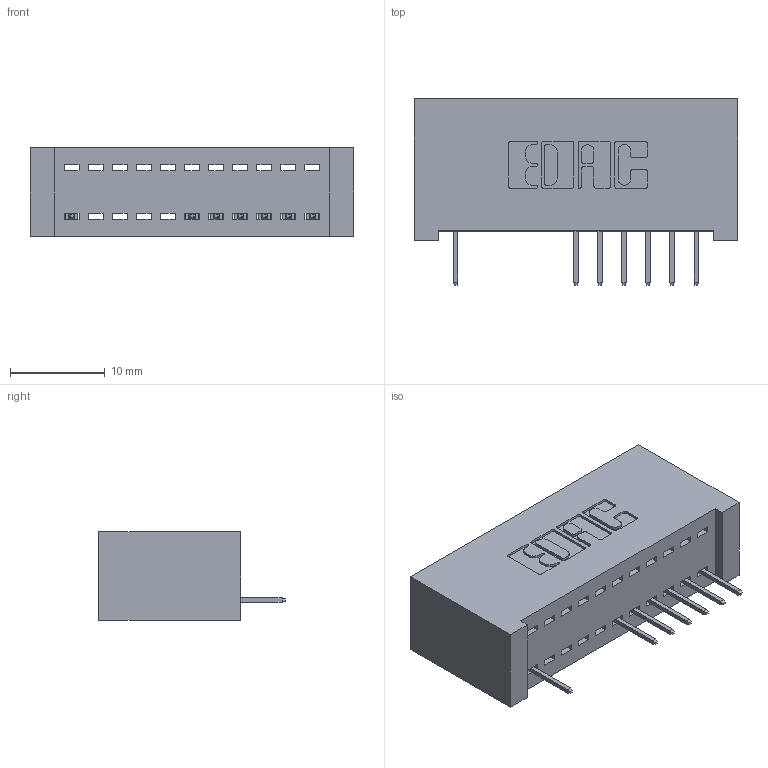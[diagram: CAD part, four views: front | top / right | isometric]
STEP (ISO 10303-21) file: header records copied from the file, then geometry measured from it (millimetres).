
FILE_DESCRIPTION (( 'STEP AP203' ), '1' );
FILE_NAME ('392-011-524-101.STEP', '2018-08-14T21:15:50', ( '' ), ( '' ), 'SwSTEP 2.0', 'SolidWorks 2016', '' );
FILE_SCHEMA (( 'CONFIG_CONTROL_DESIGN' ));
Length unit declared in the file: inch
Products named in the file (3): 392-011-524-101; 342 Part_Lugless; 345-292-001_345-293-124
Assembly tree (8 placements, depth 2):
  392-011-524-101
    342 Part_Lugless
    345-292-001_345-293-124  x7
Bounding box: 34.19 x 19.69 x 9.4 mm (x, y, z)
Volume: 3219 mm3; surface area: 4148.5 mm2
Topology: 8 solids, 8 shells, 584 faces, 1703 edges, 1106 vertices
Faces by surface type: plane 446, cylinder 138
Entity records: 10271 total; most frequent: CARTESIAN_POINT 1799, ORIENTED_EDGE 1750, DIRECTION 1569, EDGE_CURVE 875, VECTOR 759, LINE 759, VERTEX_POINT 578, AXIS2_PLACEMENT_3D 405
